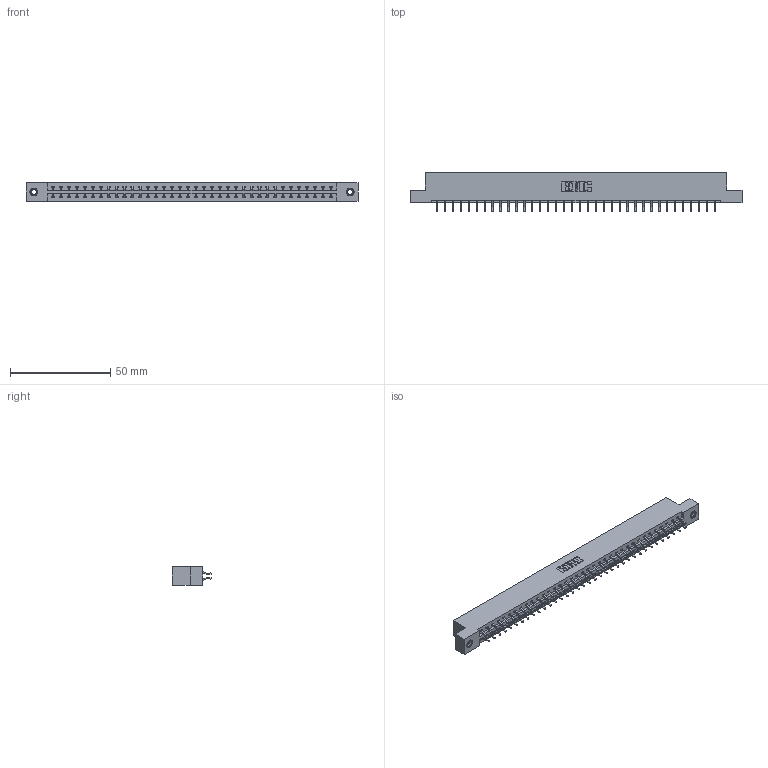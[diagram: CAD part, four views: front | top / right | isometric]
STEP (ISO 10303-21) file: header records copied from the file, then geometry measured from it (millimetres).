
FILE_DESCRIPTION (( 'STEP AP203' ), '1' );
FILE_NAME ('387-072-556-207.STEP', '2019-10-22T00:29:49', ( '' ), ( '' ), 'SwSTEP 2.0', 'SolidWorks 2016', '' );
FILE_SCHEMA (( 'CONFIG_CONTROL_DESIGN' ));
Length unit declared in the file: inch
Products named in the file (4): 337 Part_Flush Mounting Lugs - 0.156 Dia-TI; 387-072-556-207; 345-250-001_345-250-005-103; 345-292-001_556 Tail
Assembly tree (75 placements, depth 2):
  387-072-556-207
    337 Part_Flush Mounting Lugs - 0.156 Dia-TI
    345-292-001_556 Tail  x72
    345-250-001_345-250-005-103  x2
Bounding box: 165.66 x 19.57 x 9.4 mm (x, y, z)
Volume: 17362.2 mm3; surface area: 19529.7 mm2
Topology: 75 solids, 75 shells, 4494 faces, 13335 edges, 8786 vertices
Faces by surface type: plane 3126, cylinder 1352, cone 12, torus 4
Entity records: 30094 total; most frequent: CARTESIAN_POINT 5069, ORIENTED_EDGE 4986, DIRECTION 4343, EDGE_CURVE 2493, VECTOR 2337, LINE 2337, VERTEX_POINT 1656, AXIS2_PLACEMENT_3D 1003
